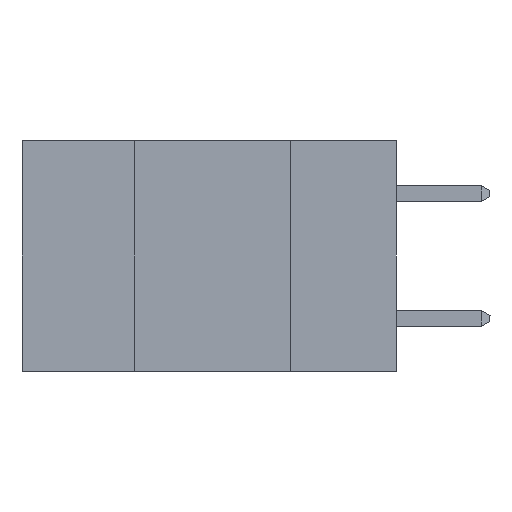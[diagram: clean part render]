
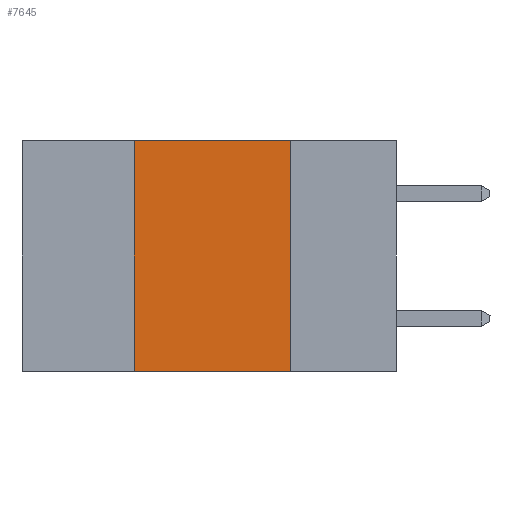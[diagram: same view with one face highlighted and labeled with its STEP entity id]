
A CAD part, left-side view. The second image highlights one B-rep face of the part: STEP entity #7645.
In plain terms, the highlighted planar face has unit normal (-1, 0, 0).
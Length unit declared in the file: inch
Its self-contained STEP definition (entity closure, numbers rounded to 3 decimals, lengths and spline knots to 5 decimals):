
#962 = DIRECTION ( 'NONE',  ( 0., 0., -1. ) ) ;
#965 = CARTESIAN_POINT ( 'NONE',  ( 0., 0.17, -0.37 ) ) ;
#1148 = CARTESIAN_POINT ( 'NONE',  ( 0., 0.6, 0. ) ) ;
#1934 = CARTESIAN_POINT ( 'NONE',  ( 0., 0.17, 0. ) ) ;
#2446 = FACE_OUTER_BOUND ( 'NONE', #12695, .T. ) ;
#3106 = DIRECTION ( 'NONE',  ( 1., 0., 0. ) ) ;
#3250 = PLANE ( 'NONE',  #14682 ) ;
#3539 = VERTEX_POINT ( 'NONE', #5943 ) ;
#4204 = LINE ( 'NONE', #10405, #13637 ) ;
#4444 = VECTOR ( 'NONE', #11164, 39.37008 ) ;
#4518 = EDGE_CURVE ( 'NONE', #5401, #3539, #12793, .T. ) ;
#5312 = EDGE_CURVE ( 'NONE', #5401, #14987, #7915, .T. ) ;
#5401 = VERTEX_POINT ( 'NONE', #9620 ) ;
#5943 = CARTESIAN_POINT ( 'NONE',  ( 0., 0.17, -0.37 ) ) ;
#6466 = DIRECTION ( 'NONE',  ( 0., 0., -1. ) ) ;
#6874 = EDGE_CURVE ( 'NONE', #14987, #8362, #4204, .T. ) ;
#7583 = ORIENTED_EDGE ( 'NONE', *, *, #5312, .F. ) ;
#7645 = ADVANCED_FACE ( 'NONE', ( #2446 ), #3250, .F. ) ;
#7656 = EDGE_CURVE ( 'NONE', #8362, #3539, #9413, .T. ) ;
#7915 = LINE ( 'NONE', #11241, #4444 ) ;
#8362 = VERTEX_POINT ( 'NONE', #1934 ) ;
#8665 = VECTOR ( 'NONE', #6466, 39.37008 ) ;
#9413 = LINE ( 'NONE', #965, #8665 ) ;
#9620 = CARTESIAN_POINT ( 'NONE',  ( 0., 0.42, -0.37 ) ) ;
#9634 = ORIENTED_EDGE ( 'NONE', *, *, #6874, .F. ) ;
#9638 = VECTOR ( 'NONE', #15380, 39.37008 ) ;
#10165 = DIRECTION ( 'NONE',  ( 0., -1., 0. ) ) ;
#10405 = CARTESIAN_POINT ( 'NONE',  ( 0., 0.6, 0. ) ) ;
#11164 = DIRECTION ( 'NONE',  ( 0., 0., 1. ) ) ;
#11241 = CARTESIAN_POINT ( 'NONE',  ( 0., 0.42, -0.37 ) ) ;
#12610 = ORIENTED_EDGE ( 'NONE', *, *, #4518, .T. ) ;
#12695 = EDGE_LOOP ( 'NONE', ( #14791, #9634, #7583, #12610 ) ) ;
#12793 = LINE ( 'NONE', #15071, #9638 ) ;
#13637 = VECTOR ( 'NONE', #10165, 39.37008 ) ;
#14198 = CARTESIAN_POINT ( 'NONE',  ( 0., 0.42, 0. ) ) ;
#14682 = AXIS2_PLACEMENT_3D ( 'NONE', #1148, #3106, #962 ) ;
#14791 = ORIENTED_EDGE ( 'NONE', *, *, #7656, .F. ) ;
#14987 = VERTEX_POINT ( 'NONE', #14198 ) ;
#15071 = CARTESIAN_POINT ( 'NONE',  ( 0., 0.6, -0.37 ) ) ;
#15380 = DIRECTION ( 'NONE',  ( 0., -1., 0. ) ) ;
